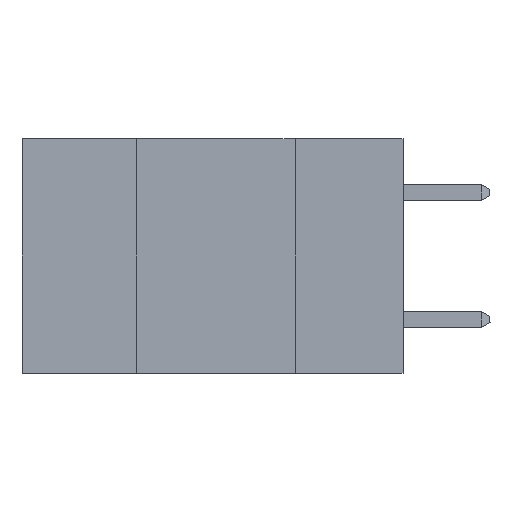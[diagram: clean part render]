
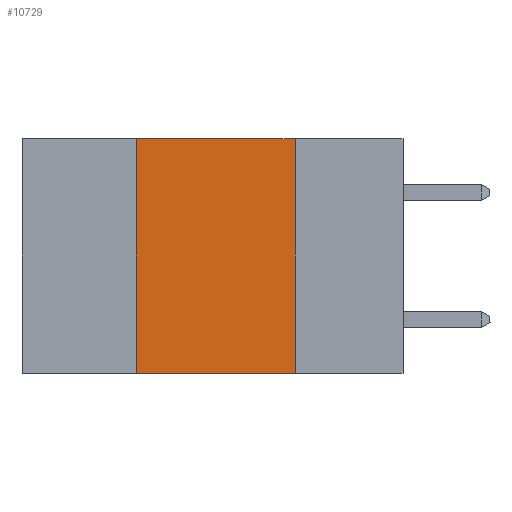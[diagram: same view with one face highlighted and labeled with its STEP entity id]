
A CAD part, left-side view. The second image highlights one B-rep face of the part: STEP entity #10729.
In plain terms, the highlighted planar face has unit normal (-1, 0, 0).
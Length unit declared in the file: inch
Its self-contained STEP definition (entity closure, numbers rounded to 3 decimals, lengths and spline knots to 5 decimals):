
#966 = EDGE_CURVE ( 'NONE', #18955, #2625, #3578, .T. ) ;
#1040 = ORIENTED_EDGE ( 'NONE', *, *, #13795, .F. ) ;
#2181 = FACE_OUTER_BOUND ( 'NONE', #18477, .T. ) ;
#2522 = CARTESIAN_POINT ( 'NONE',  ( 0., 0.6, 0. ) ) ;
#2625 = VERTEX_POINT ( 'NONE', #23785 ) ;
#3578 = LINE ( 'NONE', #17326, #5971 ) ;
#4185 = CARTESIAN_POINT ( 'NONE',  ( 0., 0.42, -0.37 ) ) ;
#4366 = VERTEX_POINT ( 'NONE', #24050 ) ;
#4473 = DIRECTION ( 'NONE',  ( 0., 0., -1. ) ) ;
#5468 = DIRECTION ( 'NONE',  ( 0., -1., 0. ) ) ;
#5649 = LINE ( 'NONE', #23164, #13086 ) ;
#5971 = VECTOR ( 'NONE', #5468, 39.37008 ) ;
#6609 = ORIENTED_EDGE ( 'NONE', *, *, #18166, .F. ) ;
#6954 = VECTOR ( 'NONE', #21917, 39.37008 ) ;
#7730 = ORIENTED_EDGE ( 'NONE', *, *, #966, .T. ) ;
#8854 = ORIENTED_EDGE ( 'NONE', *, *, #11422, .F. ) ;
#10729 = ADVANCED_FACE ( 'NONE', ( #2181 ), #15950, .F. ) ;
#11422 = EDGE_CURVE ( 'NONE', #18955, #17372, #16784, .T. ) ;
#11753 = DIRECTION ( 'NONE',  ( 1., 0., 0. ) ) ;
#13086 = VECTOR ( 'NONE', #21866, 39.37008 ) ;
#13795 = EDGE_CURVE ( 'NONE', #4366, #2625, #5649, .T. ) ;
#14340 = DIRECTION ( 'NONE',  ( 0., 0., 1. ) ) ;
#15950 = PLANE ( 'NONE',  #20107 ) ;
#16784 = LINE ( 'NONE', #18053, #22187 ) ;
#17326 = CARTESIAN_POINT ( 'NONE',  ( 0., 0.6, -0.37 ) ) ;
#17372 = VERTEX_POINT ( 'NONE', #17508 ) ;
#17508 = CARTESIAN_POINT ( 'NONE',  ( 0., 0.42, 0. ) ) ;
#18053 = CARTESIAN_POINT ( 'NONE',  ( 0., 0.42, 0. ) ) ;
#18166 = EDGE_CURVE ( 'NONE', #17372, #4366, #21879, .T. ) ;
#18477 = EDGE_LOOP ( 'NONE', ( #1040, #6609, #8854, #7730 ) ) ;
#18955 = VERTEX_POINT ( 'NONE', #4185 ) ;
#19794 = CARTESIAN_POINT ( 'NONE',  ( 0., 0.6, 0. ) ) ;
#20107 = AXIS2_PLACEMENT_3D ( 'NONE', #2522, #11753, #4473 ) ;
#21866 = DIRECTION ( 'NONE',  ( 0., 0., -1. ) ) ;
#21879 = LINE ( 'NONE', #19794, #6954 ) ;
#21917 = DIRECTION ( 'NONE',  ( 0., -1., 0. ) ) ;
#22187 = VECTOR ( 'NONE', #14340, 39.37008 ) ;
#23164 = CARTESIAN_POINT ( 'NONE',  ( 0., 0.17, 0. ) ) ;
#23785 = CARTESIAN_POINT ( 'NONE',  ( 0., 0.17, -0.37 ) ) ;
#24050 = CARTESIAN_POINT ( 'NONE',  ( 0., 0.17, 0. ) ) ;
